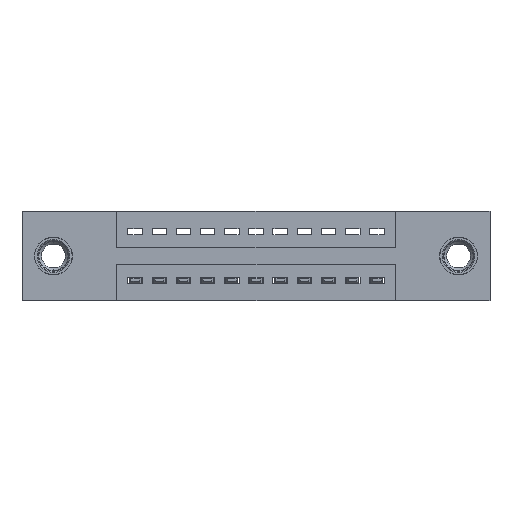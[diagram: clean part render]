
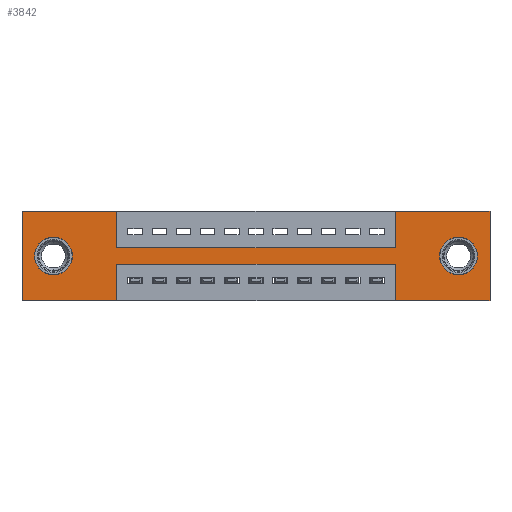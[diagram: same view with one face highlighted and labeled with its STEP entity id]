
A CAD part, front view. The second image highlights one B-rep face of the part: STEP entity #3842.
In plain terms, the highlighted planar face has unit normal (0, -1, 0).
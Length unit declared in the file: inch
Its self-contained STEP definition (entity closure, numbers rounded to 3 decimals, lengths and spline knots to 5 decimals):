
#39 = LINE ( 'NONE', #6039, #11940 ) ;
#72 = CARTESIAN_POINT ( 'NONE',  ( 1.805, 0., -0.185 ) ) ;
#121 = VERTEX_POINT ( 'NONE', #8112 ) ;
#161 = VERTEX_POINT ( 'NONE', #9365 ) ;
#195 = CARTESIAN_POINT ( 'NONE',  ( 0.3925, 0., -0.37 ) ) ;
#593 = AXIS2_PLACEMENT_3D ( 'NONE', #11022, #4763, #12095 ) ;
#654 = DIRECTION ( 'NONE',  ( 0., 1., 0. ) ) ;
#717 = DIRECTION ( 'NONE',  ( 0., 0., -1. ) ) ;
#851 = LINE ( 'NONE', #1368, #7052 ) ;
#961 = EDGE_CURVE ( 'NONE', #9235, #12820, #3203, .T. ) ;
#982 = DIRECTION ( 'NONE',  ( 0., 0., -1. ) ) ;
#1016 = CARTESIAN_POINT ( 'NONE',  ( 0.13, 0., -0.185 ) ) ;
#1184 = LINE ( 'NONE', #4312, #6397 ) ;
#1368 = CARTESIAN_POINT ( 'NONE',  ( 0., 0., 0. ) ) ;
#1731 = CARTESIAN_POINT ( 'NONE',  ( 1.935, 0., 0. ) ) ;
#1781 = CARTESIAN_POINT ( 'NONE',  ( 0.13, 0., -0.107 ) ) ;
#2157 = VECTOR ( 'NONE', #2632, 39.37008 ) ;
#2264 = DIRECTION ( 'NONE',  ( 0., 0., 1. ) ) ;
#2577 = CARTESIAN_POINT ( 'NONE',  ( 0., 0., -0.37 ) ) ;
#2632 = DIRECTION ( 'NONE',  ( 1., 0., 0. ) ) ;
#2694 = EDGE_CURVE ( 'NONE', #9179, #12608, #7249, .T. ) ;
#2740 = CARTESIAN_POINT ( 'NONE',  ( 0., 0., -0.37 ) ) ;
#3051 = VECTOR ( 'NONE', #5954, 39.37008 ) ;
#3052 = VERTEX_POINT ( 'NONE', #1781 ) ;
#3098 = EDGE_CURVE ( 'NONE', #12608, #9179, #3617, .T. ) ;
#3203 = LINE ( 'NONE', #3418, #12039 ) ;
#3248 = AXIS2_PLACEMENT_3D ( 'NONE', #1016, #11562, #10386 ) ;
#3269 = DIRECTION ( 'NONE',  ( -1., 0., 0. ) ) ;
#3395 = ORIENTED_EDGE ( 'NONE', *, *, #8214, .F. ) ;
#3409 = CARTESIAN_POINT ( 'NONE',  ( 1.935, 0., -0.37 ) ) ;
#3418 = CARTESIAN_POINT ( 'NONE',  ( 0.3925, 0., 0. ) ) ;
#3480 = ORIENTED_EDGE ( 'NONE', *, *, #11383, .F. ) ;
#3617 = CIRCLE ( 'NONE', #593, 0.078 ) ;
#3647 = LINE ( 'NONE', #7550, #5779 ) ;
#3842 = ADVANCED_FACE ( 'NONE', ( #3917, #6579, #5892 ), #5930, .T. ) ;
#3890 = CARTESIAN_POINT ( 'NONE',  ( 1.5425, 0., -0.15 ) ) ;
#3917 = FACE_BOUND ( 'NONE', #11361, .T. ) ;
#3997 = CARTESIAN_POINT ( 'NONE',  ( 0.3925, 0., 0. ) ) ;
#4010 = LINE ( 'NONE', #195, #11567 ) ;
#4312 = CARTESIAN_POINT ( 'NONE',  ( 0., 0., -0.37 ) ) ;
#4339 = EDGE_CURVE ( 'NONE', #8090, #13426, #1184, .T. ) ;
#4393 = CARTESIAN_POINT ( 'NONE',  ( 1.5425, 0., -0.37 ) ) ;
#4652 = ORIENTED_EDGE ( 'NONE', *, *, #10295, .F. ) ;
#4667 = CIRCLE ( 'NONE', #3248, 0.078 ) ;
#4747 = CARTESIAN_POINT ( 'NONE',  ( 1.805, 0., -0.107 ) ) ;
#4763 = DIRECTION ( 'NONE',  ( 0., 1., 0. ) ) ;
#4917 = ORIENTED_EDGE ( 'NONE', *, *, #6582, .T. ) ;
#5205 = CARTESIAN_POINT ( 'NONE',  ( 0.13, 0., -0.263 ) ) ;
#5391 = ORIENTED_EDGE ( 'NONE', *, *, #9994, .F. ) ;
#5428 = VERTEX_POINT ( 'NONE', #6259 ) ;
#5485 = LINE ( 'NONE', #13093, #12193 ) ;
#5561 = ORIENTED_EDGE ( 'NONE', *, *, #5884, .F. ) ;
#5594 = DIRECTION ( 'NONE',  ( 1., 0., 0. ) ) ;
#5711 = EDGE_CURVE ( 'NONE', #12820, #10310, #7728, .T. ) ;
#5779 = VECTOR ( 'NONE', #12812, 39.37008 ) ;
#5884 = EDGE_CURVE ( 'NONE', #11980, #11846, #12766, .T. ) ;
#5892 = FACE_OUTER_BOUND ( 'NONE', #8129, .T. ) ;
#5930 = PLANE ( 'NONE',  #10480 ) ;
#5954 = DIRECTION ( 'NONE',  ( 0., 0., 1. ) ) ;
#6039 = CARTESIAN_POINT ( 'NONE',  ( 0., 0., -0.37 ) ) ;
#6065 = VERTEX_POINT ( 'NONE', #5205 ) ;
#6076 = ORIENTED_EDGE ( 'NONE', *, *, #3098, .T. ) ;
#6259 = CARTESIAN_POINT ( 'NONE',  ( 1.5425, 0., -0.22 ) ) ;
#6285 = EDGE_CURVE ( 'NONE', #161, #9235, #851, .T. ) ;
#6289 = CARTESIAN_POINT ( 'NONE',  ( 0.3925, 0., -0.22 ) ) ;
#6397 = VECTOR ( 'NONE', #3269, 39.37008 ) ;
#6513 = EDGE_CURVE ( 'NONE', #11846, #8899, #39, .T. ) ;
#6535 = CARTESIAN_POINT ( 'NONE',  ( 0.3925, 0., -0.15 ) ) ;
#6579 = FACE_BOUND ( 'NONE', #7314, .T. ) ;
#6582 = EDGE_CURVE ( 'NONE', #3052, #6065, #12588, .T. ) ;
#6584 = DIRECTION ( 'NONE',  ( 0., 0., -1. ) ) ;
#6731 = CARTESIAN_POINT ( 'NONE',  ( 0.3925, 0., -0.15 ) ) ;
#7052 = VECTOR ( 'NONE', #5594, 39.37008 ) ;
#7225 = DIRECTION ( 'NONE',  ( 0., 1., 0. ) ) ;
#7249 = CIRCLE ( 'NONE', #13150, 0.078 ) ;
#7314 = EDGE_LOOP ( 'NONE', ( #4917, #11590 ) ) ;
#7550 = CARTESIAN_POINT ( 'NONE',  ( 0.3925, 0., -0.22 ) ) ;
#7689 = ORIENTED_EDGE ( 'NONE', *, *, #6285, .F. ) ;
#7728 = LINE ( 'NONE', #6731, #2157 ) ;
#7771 = VECTOR ( 'NONE', #11735, 39.37008 ) ;
#8090 = VERTEX_POINT ( 'NONE', #10592 ) ;
#8112 = CARTESIAN_POINT ( 'NONE',  ( 1.5425, 0., 0. ) ) ;
#8129 = EDGE_LOOP ( 'NONE', ( #3395, #4652, #3480, #13222, #5561, #8818, #12613, #12823, #11235, #7689, #5391, #12514 ) ) ;
#8214 = EDGE_CURVE ( 'NONE', #9545, #8090, #4010, .T. ) ;
#8818 = ORIENTED_EDGE ( 'NONE', *, *, #13402, .F. ) ;
#8899 = VERTEX_POINT ( 'NONE', #4393 ) ;
#8978 = DIRECTION ( 'NONE',  ( 1., 0., 0. ) ) ;
#9017 = VECTOR ( 'NONE', #12057, 39.37008 ) ;
#9074 = LINE ( 'NONE', #9806, #7771 ) ;
#9127 = CARTESIAN_POINT ( 'NONE',  ( 1.805, 0., -0.263 ) ) ;
#9179 = VERTEX_POINT ( 'NONE', #4747 ) ;
#9235 = VERTEX_POINT ( 'NONE', #3997 ) ;
#9365 = CARTESIAN_POINT ( 'NONE',  ( 0., 0., 0. ) ) ;
#9433 = DIRECTION ( 'NONE',  ( 0., 0., -1. ) ) ;
#9545 = VERTEX_POINT ( 'NONE', #6289 ) ;
#9806 = CARTESIAN_POINT ( 'NONE',  ( 0., 0., 0. ) ) ;
#9955 = CARTESIAN_POINT ( 'NONE',  ( 1.5425, 0., 0. ) ) ;
#9994 = EDGE_CURVE ( 'NONE', #13426, #161, #9074, .T. ) ;
#10033 = DIRECTION ( 'NONE',  ( 0., 0., 1. ) ) ;
#10295 = EDGE_CURVE ( 'NONE', #5428, #9545, #3647, .T. ) ;
#10310 = VERTEX_POINT ( 'NONE', #3890 ) ;
#10386 = DIRECTION ( 'NONE',  ( 0., 0., 1. ) ) ;
#10480 = AXIS2_PLACEMENT_3D ( 'NONE', #2740, #11105, #717 ) ;
#10592 = CARTESIAN_POINT ( 'NONE',  ( 0.3925, 0., -0.37 ) ) ;
#10702 = CARTESIAN_POINT ( 'NONE',  ( 1.5425, 0., -0.37 ) ) ;
#10945 = CARTESIAN_POINT ( 'NONE',  ( 1.935, 0., 0. ) ) ;
#11010 = AXIS2_PLACEMENT_3D ( 'NONE', #12059, #654, #10033 ) ;
#11022 = CARTESIAN_POINT ( 'NONE',  ( 1.805, 0., -0.185 ) ) ;
#11105 = DIRECTION ( 'NONE',  ( 0., -1., 0. ) ) ;
#11235 = ORIENTED_EDGE ( 'NONE', *, *, #961, .F. ) ;
#11361 = EDGE_LOOP ( 'NONE', ( #11865, #6076 ) ) ;
#11383 = EDGE_CURVE ( 'NONE', #8899, #5428, #11611, .T. ) ;
#11562 = DIRECTION ( 'NONE',  ( 0., 1., 0. ) ) ;
#11567 = VECTOR ( 'NONE', #9433, 39.37008 ) ;
#11590 = ORIENTED_EDGE ( 'NONE', *, *, #13066, .T. ) ;
#11611 = LINE ( 'NONE', #10702, #13038 ) ;
#11735 = DIRECTION ( 'NONE',  ( 0., 0., 1. ) ) ;
#11846 = VERTEX_POINT ( 'NONE', #3409 ) ;
#11865 = ORIENTED_EDGE ( 'NONE', *, *, #2694, .T. ) ;
#11940 = VECTOR ( 'NONE', #12179, 39.37008 ) ;
#11980 = VERTEX_POINT ( 'NONE', #10945 ) ;
#12039 = VECTOR ( 'NONE', #6584, 39.37008 ) ;
#12057 = DIRECTION ( 'NONE',  ( 0., 0., -1. ) ) ;
#12059 = CARTESIAN_POINT ( 'NONE',  ( 0.13, 0., -0.185 ) ) ;
#12095 = DIRECTION ( 'NONE',  ( 0., 0., -1. ) ) ;
#12179 = DIRECTION ( 'NONE',  ( -1., 0., 0. ) ) ;
#12193 = VECTOR ( 'NONE', #8978, 39.37008 ) ;
#12514 = ORIENTED_EDGE ( 'NONE', *, *, #4339, .F. ) ;
#12526 = EDGE_CURVE ( 'NONE', #10310, #121, #12547, .T. ) ;
#12547 = LINE ( 'NONE', #9955, #3051 ) ;
#12588 = CIRCLE ( 'NONE', #11010, 0.078 ) ;
#12608 = VERTEX_POINT ( 'NONE', #9127 ) ;
#12613 = ORIENTED_EDGE ( 'NONE', *, *, #12526, .F. ) ;
#12766 = LINE ( 'NONE', #1731, #9017 ) ;
#12812 = DIRECTION ( 'NONE',  ( -1., 0., 0. ) ) ;
#12820 = VERTEX_POINT ( 'NONE', #6535 ) ;
#12823 = ORIENTED_EDGE ( 'NONE', *, *, #5711, .F. ) ;
#13038 = VECTOR ( 'NONE', #2264, 39.37008 ) ;
#13066 = EDGE_CURVE ( 'NONE', #6065, #3052, #4667, .T. ) ;
#13093 = CARTESIAN_POINT ( 'NONE',  ( 0., 0., 0. ) ) ;
#13150 = AXIS2_PLACEMENT_3D ( 'NONE', #72, #7225, #982 ) ;
#13222 = ORIENTED_EDGE ( 'NONE', *, *, #6513, .F. ) ;
#13402 = EDGE_CURVE ( 'NONE', #121, #11980, #5485, .T. ) ;
#13426 = VERTEX_POINT ( 'NONE', #2577 ) ;
